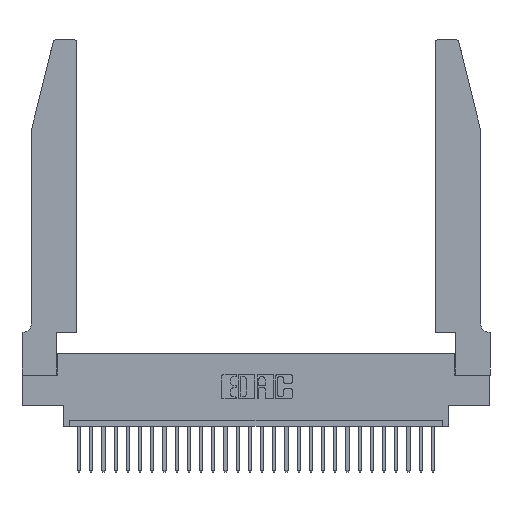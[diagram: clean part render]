
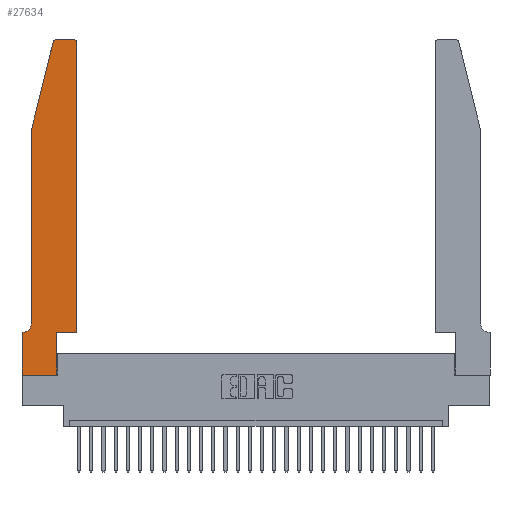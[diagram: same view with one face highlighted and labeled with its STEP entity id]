
A CAD part, top view. The second image highlights one B-rep face of the part: STEP entity #27634.
In plain terms, the highlighted planar face has unit normal (0, 0, 1).
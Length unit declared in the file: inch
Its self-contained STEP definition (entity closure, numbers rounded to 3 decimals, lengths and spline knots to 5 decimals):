
#8 = ORIENTED_EDGE ( 'NONE', *, *, #22802, .T. ) ;
#179 = CARTESIAN_POINT ( 'NONE',  ( 0.4205, 2.72, 0.37 ) ) ;
#446 = DIRECTION ( 'NONE',  ( 0., -1., 0. ) ) ;
#1122 = DIRECTION ( 'NONE',  ( 0., -1., 0. ) ) ;
#1224 = EDGE_CURVE ( 'NONE', #28636, #19274, #24081, .T. ) ;
#1289 = LINE ( 'NONE', #16451, #5850 ) ;
#1517 = CARTESIAN_POINT ( 'NONE',  ( 0.2865, 0., 0.37 ) ) ;
#1638 = EDGE_CURVE ( 'NONE', #21732, #4862, #3983, .T. ) ;
#1834 = CARTESIAN_POINT ( 'NONE',  ( 0.25487, 2.72718, 0.37 ) ) ;
#3204 = ORIENTED_EDGE ( 'NONE', *, *, #7960, .T. ) ;
#3387 = DIRECTION ( 'NONE',  ( 0., 0., 1. ) ) ;
#3983 = LINE ( 'NONE', #9043, #12792 ) ;
#4377 = CARTESIAN_POINT ( 'NONE',  ( 0.4505, 2.72, 0.37 ) ) ;
#4717 = ORIENTED_EDGE ( 'NONE', *, *, #16930, .T. ) ;
#4745 = DIRECTION ( 'NONE',  ( 1., 0., 0. ) ) ;
#4862 = VERTEX_POINT ( 'NONE', #5584 ) ;
#5584 = CARTESIAN_POINT ( 'NONE',  ( 0.4505, 0.35, 0.37 ) ) ;
#5850 = VECTOR ( 'NONE', #7793, 39.37008 ) ;
#6126 = DIRECTION ( 'NONE',  ( 0., 0., -1. ) ) ;
#6134 = VECTOR ( 'NONE', #16313, 39.37008 ) ;
#6304 = VERTEX_POINT ( 'NONE', #1517 ) ;
#7459 = VECTOR ( 'NONE', #20272, 39.37008 ) ;
#7793 = DIRECTION ( 'NONE',  ( 0., 1., 0. ) ) ;
#7917 = ORIENTED_EDGE ( 'NONE', *, *, #9705, .T. ) ;
#7960 = EDGE_CURVE ( 'NONE', #19274, #27735, #11731, .T. ) ;
#8112 = VERTEX_POINT ( 'NONE', #4377 ) ;
#8298 = VERTEX_POINT ( 'NONE', #25936 ) ;
#8405 = VERTEX_POINT ( 'NONE', #1834 ) ;
#8852 = DIRECTION ( 'NONE',  ( 1., 0., 0. ) ) ;
#9043 = CARTESIAN_POINT ( 'NONE',  ( 0.4505, 0.35, 0.37 ) ) ;
#9705 = EDGE_CURVE ( 'NONE', #8112, #23801, #14437, .T. ) ;
#9718 = CARTESIAN_POINT ( 'NONE',  ( 0.0055, 0.35, 0.37 ) ) ;
#10478 = VECTOR ( 'NONE', #17653, 39.37008 ) ;
#11179 = LINE ( 'NONE', #26842, #10478 ) ;
#11580 = CIRCLE ( 'NONE', #24399, 0.03 ) ;
#11731 = LINE ( 'NONE', #16470, #19471 ) ;
#11869 = DIRECTION ( 'NONE',  ( 0., 0., 1. ) ) ;
#12024 = FACE_OUTER_BOUND ( 'NONE', #23910, .T. ) ;
#12406 = ORIENTED_EDGE ( 'NONE', *, *, #19537, .T. ) ;
#12601 = DIRECTION ( 'NONE',  ( -0.239, -0.971, 0. ) ) ;
#12792 = VECTOR ( 'NONE', #8852, 39.37008 ) ;
#13639 = ORIENTED_EDGE ( 'NONE', *, *, #15942, .T. ) ;
#13746 = CARTESIAN_POINT ( 'NONE',  ( 0.4205, 2.75, 0.37 ) ) ;
#13819 = DIRECTION ( 'NONE',  ( 0., 0., 1. ) ) ;
#14437 = CIRCLE ( 'NONE', #18350, 0.03 ) ;
#14651 = CARTESIAN_POINT ( 'NONE',  ( 0.0755, 2., 0.37 ) ) ;
#15160 = CARTESIAN_POINT ( 'NONE',  ( 0., 0., 0.37 ) ) ;
#15462 = ORIENTED_EDGE ( 'NONE', *, *, #21746, .T. ) ;
#15942 = EDGE_CURVE ( 'NONE', #23801, #26024, #17285, .T. ) ;
#15967 = CARTESIAN_POINT ( 'NONE',  ( 0.284, 2.72, 0.37 ) ) ;
#16068 = CARTESIAN_POINT ( 'NONE',  ( 0.0755, 2., 0.37 ) ) ;
#16101 = DIRECTION ( 'NONE',  ( 1., 0., 0. ) ) ;
#16105 = CARTESIAN_POINT ( 'NONE',  ( 0.0755, 0.35, 0.37 ) ) ;
#16313 = DIRECTION ( 'NONE',  ( -1., 0., 0. ) ) ;
#16451 = CARTESIAN_POINT ( 'NONE',  ( 0.2865, 0.35, 0.37 ) ) ;
#16470 = CARTESIAN_POINT ( 'NONE',  ( 0., 0., 0.37 ) ) ;
#16620 = ORIENTED_EDGE ( 'NONE', *, *, #17331, .T. ) ;
#16864 = CARTESIAN_POINT ( 'NONE',  ( 0., 0.35, 0.37 ) ) ;
#16930 = EDGE_CURVE ( 'NONE', #8405, #8298, #21740, .T. ) ;
#17259 = ORIENTED_EDGE ( 'NONE', *, *, #17618, .T. ) ;
#17285 = LINE ( 'NONE', #26721, #24639 ) ;
#17331 = EDGE_CURVE ( 'NONE', #21449, #28636, #23867, .T. ) ;
#17425 = LINE ( 'NONE', #16068, #24786 ) ;
#17501 = ORIENTED_EDGE ( 'NONE', *, *, #1224, .T. ) ;
#17618 = EDGE_CURVE ( 'NONE', #4862, #8112, #26102, .T. ) ;
#17653 = DIRECTION ( 'NONE',  ( 1., 0., 0. ) ) ;
#18193 = CARTESIAN_POINT ( 'NONE',  ( 0.0755, 0.42, 0.37 ) ) ;
#18350 = AXIS2_PLACEMENT_3D ( 'NONE', #179, #13819, #16101 ) ;
#19274 = VERTEX_POINT ( 'NONE', #24209 ) ;
#19386 = DIRECTION ( 'NONE',  ( -1., 0., 0. ) ) ;
#19444 = AXIS2_PLACEMENT_3D ( 'NONE', #16864, #3387, #28129 ) ;
#19471 = VECTOR ( 'NONE', #1122, 39.37008 ) ;
#19493 = PLANE ( 'NONE',  #19444 ) ;
#19537 = EDGE_CURVE ( 'NONE', #26024, #8405, #11580, .T. ) ;
#19668 = ORIENTED_EDGE ( 'NONE', *, *, #1638, .T. ) ;
#20272 = DIRECTION ( 'NONE',  ( 0., 1., 0. ) ) ;
#21177 = CARTESIAN_POINT ( 'NONE',  ( 0.4505, 0.35, 0.37 ) ) ;
#21449 = VERTEX_POINT ( 'NONE', #18193 ) ;
#21732 = VERTEX_POINT ( 'NONE', #24808 ) ;
#21740 = LINE ( 'NONE', #14651, #28805 ) ;
#21746 = EDGE_CURVE ( 'NONE', #27735, #6304, #11179, .T. ) ;
#21945 = CARTESIAN_POINT ( 'NONE',  ( 0.284, 2.75, 0.37 ) ) ;
#22062 = EDGE_CURVE ( 'NONE', #6304, #21732, #1289, .T. ) ;
#22401 = DIRECTION ( 'NONE',  ( -1., 0., 0. ) ) ;
#22802 = EDGE_CURVE ( 'NONE', #8298, #21449, #17425, .T. ) ;
#22815 = AXIS2_PLACEMENT_3D ( 'NONE', #28327, #6126, #19386 ) ;
#23801 = VERTEX_POINT ( 'NONE', #13746 ) ;
#23867 = CIRCLE ( 'NONE', #22815, 0.07 ) ;
#23910 = EDGE_LOOP ( 'NONE', ( #13639, #12406, #4717, #8, #16620, #17501, #3204, #15462, #25708, #19668, #17259, #7917 ) ) ;
#24081 = LINE ( 'NONE', #16105, #6134 ) ;
#24209 = CARTESIAN_POINT ( 'NONE',  ( 0., 0.35, 0.37 ) ) ;
#24399 = AXIS2_PLACEMENT_3D ( 'NONE', #15967, #11869, #4745 ) ;
#24639 = VECTOR ( 'NONE', #22401, 39.37008 ) ;
#24786 = VECTOR ( 'NONE', #446, 39.37008 ) ;
#24808 = CARTESIAN_POINT ( 'NONE',  ( 0.2865, 0.35, 0.37 ) ) ;
#25708 = ORIENTED_EDGE ( 'NONE', *, *, #22062, .T. ) ;
#25936 = CARTESIAN_POINT ( 'NONE',  ( 0.0755, 2., 0.37 ) ) ;
#26024 = VERTEX_POINT ( 'NONE', #21945 ) ;
#26102 = LINE ( 'NONE', #21177, #7459 ) ;
#26721 = CARTESIAN_POINT ( 'NONE',  ( 0.2605, 2.75, 0.37 ) ) ;
#26842 = CARTESIAN_POINT ( 'NONE',  ( 0., 0., 0.37 ) ) ;
#27634 = ADVANCED_FACE ( 'NONE', ( #12024 ), #19493, .T. ) ;
#27735 = VERTEX_POINT ( 'NONE', #15160 ) ;
#28129 = DIRECTION ( 'NONE',  ( 1., 0., 0. ) ) ;
#28327 = CARTESIAN_POINT ( 'NONE',  ( 0.0055, 0.42, 0.37 ) ) ;
#28636 = VERTEX_POINT ( 'NONE', #9718 ) ;
#28805 = VECTOR ( 'NONE', #12601, 39.37008 ) ;
